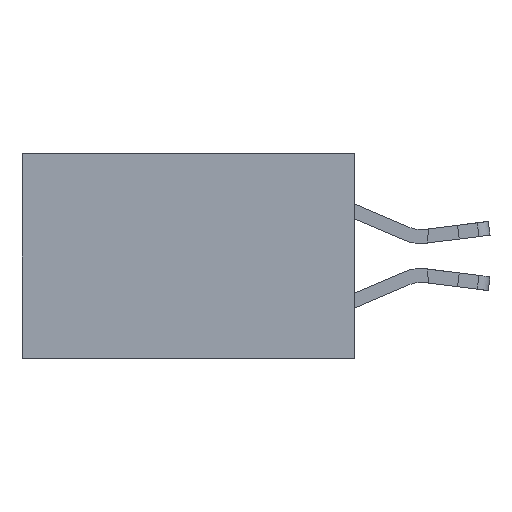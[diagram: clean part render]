
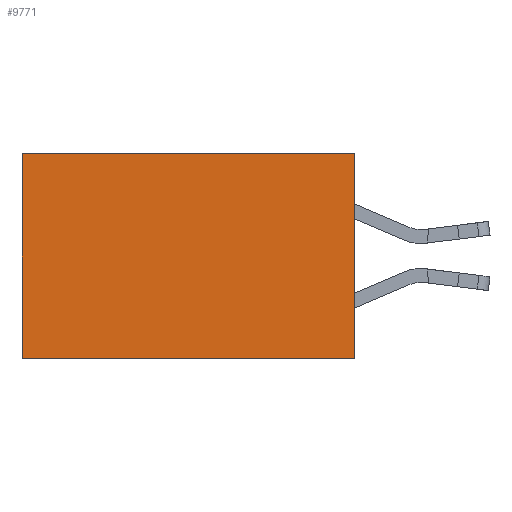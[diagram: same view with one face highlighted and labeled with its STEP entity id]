
A CAD part, left-side view. The second image highlights one B-rep face of the part: STEP entity #9771.
In plain terms, the highlighted planar face has unit normal (-1, 0, 0).
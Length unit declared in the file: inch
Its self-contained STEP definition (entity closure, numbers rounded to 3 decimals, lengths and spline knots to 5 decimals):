
#655 = VECTOR ( 'NONE', #9136, 39.37008 ) ;
#810 = CARTESIAN_POINT ( 'NONE',  ( 0.2615, 0., -0.37 ) ) ;
#1023 = LINE ( 'NONE', #5256, #4095 ) ;
#1772 = LINE ( 'NONE', #4257, #7149 ) ;
#2005 = EDGE_CURVE ( 'NONE', #12304, #4891, #4884, .T. ) ;
#2354 = DIRECTION ( 'NONE',  ( 0., 1., 0. ) ) ;
#3019 = EDGE_LOOP ( 'NONE', ( #10514, #3121, #5312, #8356 ) ) ;
#3118 = VERTEX_POINT ( 'NONE', #9175 ) ;
#3121 = ORIENTED_EDGE ( 'NONE', *, *, #9121, .F. ) ;
#4095 = VECTOR ( 'NONE', #9584, 39.37008 ) ;
#4257 = CARTESIAN_POINT ( 'NONE',  ( 0.2615, 0., 0. ) ) ;
#4884 = LINE ( 'NONE', #5782, #655 ) ;
#4891 = VERTEX_POINT ( 'NONE', #7318 ) ;
#5040 = DIRECTION ( 'NONE',  ( 1., 0., 0. ) ) ;
#5174 = PLANE ( 'NONE',  #13064 ) ;
#5246 = DIRECTION ( 'NONE',  ( 0., 0., -1. ) ) ;
#5256 = CARTESIAN_POINT ( 'NONE',  ( 0.2615, 0.6, -0.37 ) ) ;
#5312 = ORIENTED_EDGE ( 'NONE', *, *, #2005, .F. ) ;
#5782 = CARTESIAN_POINT ( 'NONE',  ( 0.2615, 0., -0.37 ) ) ;
#6312 = EDGE_CURVE ( 'NONE', #10277, #3118, #1023, .T. ) ;
#7111 = CARTESIAN_POINT ( 'NONE',  ( 0.2615, 0.6, 0. ) ) ;
#7149 = VECTOR ( 'NONE', #7382, 39.37008 ) ;
#7318 = CARTESIAN_POINT ( 'NONE',  ( 0.2615, 0., -0.37 ) ) ;
#7382 = DIRECTION ( 'NONE',  ( 0., 1., 0. ) ) ;
#7620 = LINE ( 'NONE', #11904, #10174 ) ;
#8356 = ORIENTED_EDGE ( 'NONE', *, *, #13405, .T. ) ;
#9121 = EDGE_CURVE ( 'NONE', #4891, #3118, #7620, .T. ) ;
#9136 = DIRECTION ( 'NONE',  ( 0., 0., -1. ) ) ;
#9175 = CARTESIAN_POINT ( 'NONE',  ( 0.2615, 0.6, -0.37 ) ) ;
#9584 = DIRECTION ( 'NONE',  ( 0., 0., -1. ) ) ;
#9771 = ADVANCED_FACE ( 'NONE', ( #10412 ), #5174, .F. ) ;
#10174 = VECTOR ( 'NONE', #2354, 39.37008 ) ;
#10188 = CARTESIAN_POINT ( 'NONE',  ( 0.2615, 0., 0. ) ) ;
#10277 = VERTEX_POINT ( 'NONE', #7111 ) ;
#10412 = FACE_OUTER_BOUND ( 'NONE', #3019, .T. ) ;
#10514 = ORIENTED_EDGE ( 'NONE', *, *, #6312, .T. ) ;
#11904 = CARTESIAN_POINT ( 'NONE',  ( 0.2615, 0., -0.37 ) ) ;
#12304 = VERTEX_POINT ( 'NONE', #10188 ) ;
#13064 = AXIS2_PLACEMENT_3D ( 'NONE', #810, #5040, #5246 ) ;
#13405 = EDGE_CURVE ( 'NONE', #12304, #10277, #1772, .T. ) ;
